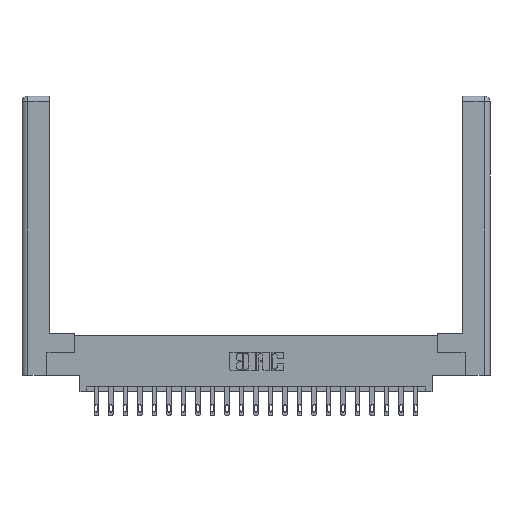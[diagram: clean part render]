
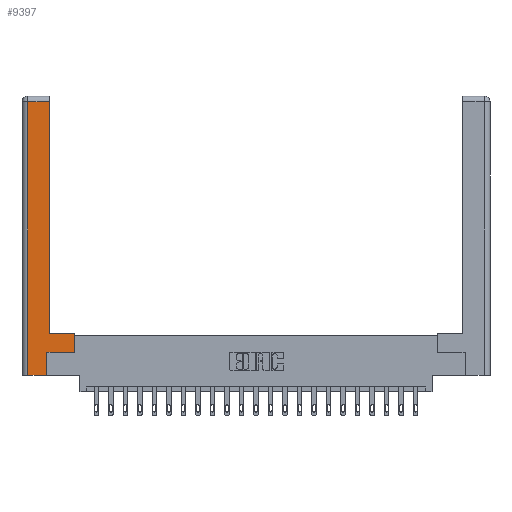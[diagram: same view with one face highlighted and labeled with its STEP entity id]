
A CAD part, top view. The second image highlights one B-rep face of the part: STEP entity #9397.
In plain terms, the highlighted planar face has unit normal (0, 0, 1).
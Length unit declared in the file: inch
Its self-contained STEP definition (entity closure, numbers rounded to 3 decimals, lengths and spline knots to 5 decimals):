
#190 = VECTOR ( 'NONE', #14046, 39.37008 ) ;
#402 = DIRECTION ( 'NONE',  ( -1., 0., 0. ) ) ;
#481 = VERTEX_POINT ( 'NONE', #14151 ) ;
#546 = CARTESIAN_POINT ( 'NONE',  ( 0.565, 0.245, 0. ) ) ;
#929 = EDGE_CURVE ( 'NONE', #481, #15108, #8092, .T. ) ;
#1315 = EDGE_CURVE ( 'NONE', #15374, #11054, #3110, .T. ) ;
#1592 = LINE ( 'NONE', #19435, #190 ) ;
#2634 = EDGE_CURVE ( 'NONE', #11054, #11686, #3045, .T. ) ;
#2640 = CARTESIAN_POINT ( 'NONE',  ( 0., 0., 0. ) ) ;
#3045 = LINE ( 'NONE', #5336, #21963 ) ;
#3048 = CARTESIAN_POINT ( 'NONE',  ( 0.0615, 0., 0. ) ) ;
#3110 = LINE ( 'NONE', #546, #21474 ) ;
#3781 = EDGE_CURVE ( 'NONE', #9100, #15374, #1592, .T. ) ;
#4017 = ORIENTED_EDGE ( 'NONE', *, *, #1315, .T. ) ;
#4288 = DIRECTION ( 'NONE',  ( -1., 0., 0. ) ) ;
#4329 = CARTESIAN_POINT ( 'NONE',  ( 0.565, 0.45, 0. ) ) ;
#4354 = DIRECTION ( 'NONE',  ( 0., 0., -1. ) ) ;
#5000 = EDGE_CURVE ( 'NONE', #15108, #7577, #8133, .T. ) ;
#5336 = CARTESIAN_POINT ( 'NONE',  ( 0.565, 0.45, 0. ) ) ;
#6440 = VECTOR ( 'NONE', #8347, 39.37008 ) ;
#6989 = ORIENTED_EDGE ( 'NONE', *, *, #13335, .T. ) ;
#7577 = VERTEX_POINT ( 'NONE', #21360 ) ;
#7875 = VECTOR ( 'NONE', #402, 39.37008 ) ;
#8092 = LINE ( 'NONE', #20909, #6440 ) ;
#8133 = LINE ( 'NONE', #14815, #7875 ) ;
#8347 = DIRECTION ( 'NONE',  ( 0., 1., 0. ) ) ;
#8434 = VECTOR ( 'NONE', #22033, 39.37008 ) ;
#8766 = FACE_OUTER_BOUND ( 'NONE', #20371, .T. ) ;
#8989 = LINE ( 'NONE', #22257, #8434 ) ;
#9100 = VERTEX_POINT ( 'NONE', #15740 ) ;
#9164 = DIRECTION ( 'NONE',  ( 0., 1., 0. ) ) ;
#9397 = ADVANCED_FACE ( 'NONE', ( #8766 ), #9666, .F. ) ;
#9561 = ORIENTED_EDGE ( 'NONE', *, *, #2634, .T. ) ;
#9666 = PLANE ( 'NONE',  #20377 ) ;
#10022 = CARTESIAN_POINT ( 'NONE',  ( 0.0615, 0., 0. ) ) ;
#11054 = VERTEX_POINT ( 'NONE', #21876 ) ;
#11355 = ORIENTED_EDGE ( 'NONE', *, *, #5000, .T. ) ;
#11686 = VERTEX_POINT ( 'NONE', #4329 ) ;
#11746 = ORIENTED_EDGE ( 'NONE', *, *, #3781, .T. ) ;
#11836 = DIRECTION ( 'NONE',  ( 0., -1., 0. ) ) ;
#12729 = ORIENTED_EDGE ( 'NONE', *, *, #929, .T. ) ;
#12893 = ORIENTED_EDGE ( 'NONE', *, *, #21119, .T. ) ;
#13279 = EDGE_CURVE ( 'NONE', #17064, #9100, #8989, .T. ) ;
#13335 = EDGE_CURVE ( 'NONE', #11686, #481, #16223, .T. ) ;
#14046 = DIRECTION ( 'NONE',  ( 0., 1., 0. ) ) ;
#14151 = CARTESIAN_POINT ( 'NONE',  ( 0.295, 0.45, 0. ) ) ;
#14607 = CARTESIAN_POINT ( 'NONE',  ( 0.295, 0.45, 0. ) ) ;
#14815 = CARTESIAN_POINT ( 'NONE',  ( 0.0615, 2.94, 0. ) ) ;
#15108 = VERTEX_POINT ( 'NONE', #22723 ) ;
#15374 = VERTEX_POINT ( 'NONE', #18653 ) ;
#15634 = VECTOR ( 'NONE', #11836, 39.37008 ) ;
#15740 = CARTESIAN_POINT ( 'NONE',  ( 0.265, 0., 0. ) ) ;
#16223 = LINE ( 'NONE', #14607, #19036 ) ;
#16471 = DIRECTION ( 'NONE',  ( -1., 0., 0. ) ) ;
#17064 = VERTEX_POINT ( 'NONE', #3048 ) ;
#17297 = DIRECTION ( 'NONE',  ( 1., 0., 0. ) ) ;
#18156 = ORIENTED_EDGE ( 'NONE', *, *, #13279, .T. ) ;
#18653 = CARTESIAN_POINT ( 'NONE',  ( 0.265, 0.245, 0. ) ) ;
#19036 = VECTOR ( 'NONE', #16471, 39.37008 ) ;
#19435 = CARTESIAN_POINT ( 'NONE',  ( 0.265, 0.245, 0. ) ) ;
#20371 = EDGE_LOOP ( 'NONE', ( #12729, #11355, #12893, #18156, #11746, #4017, #9561, #6989 ) ) ;
#20377 = AXIS2_PLACEMENT_3D ( 'NONE', #2640, #4354, #4288 ) ;
#20909 = CARTESIAN_POINT ( 'NONE',  ( 0.295, 3., 0. ) ) ;
#21119 = EDGE_CURVE ( 'NONE', #7577, #17064, #22062, .T. ) ;
#21360 = CARTESIAN_POINT ( 'NONE',  ( 0.0615, 2.94, 0. ) ) ;
#21474 = VECTOR ( 'NONE', #17297, 39.37008 ) ;
#21876 = CARTESIAN_POINT ( 'NONE',  ( 0.565, 0.245, 0. ) ) ;
#21963 = VECTOR ( 'NONE', #9164, 39.37008 ) ;
#22033 = DIRECTION ( 'NONE',  ( 1., 0., 0. ) ) ;
#22062 = LINE ( 'NONE', #10022, #15634 ) ;
#22257 = CARTESIAN_POINT ( 'NONE',  ( 0.265, 0., 0. ) ) ;
#22723 = CARTESIAN_POINT ( 'NONE',  ( 0.295, 2.94, 0. ) ) ;
